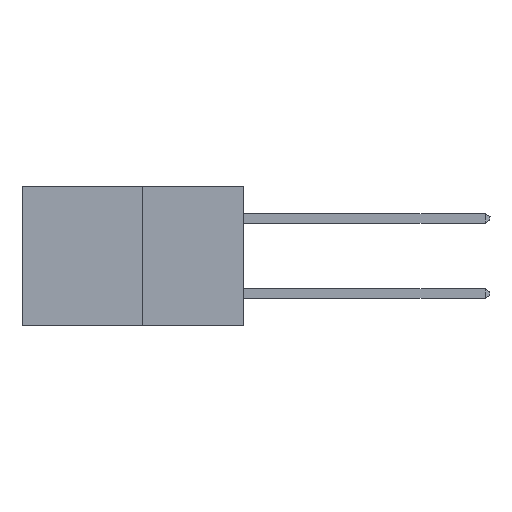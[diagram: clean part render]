
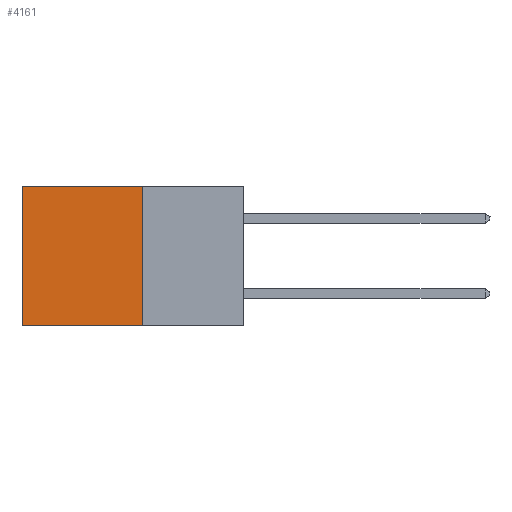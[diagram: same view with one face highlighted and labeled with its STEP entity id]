
A CAD part, left-side view. The second image highlights one B-rep face of the part: STEP entity #4161.
In plain terms, the highlighted planar face has unit normal (-1, 0, 0).
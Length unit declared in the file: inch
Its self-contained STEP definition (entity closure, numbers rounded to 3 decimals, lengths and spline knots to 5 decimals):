
#48 = CARTESIAN_POINT ( 'NONE',  ( 0.277, 0.59, -0.37 ) ) ;
#513 = EDGE_CURVE ( 'NONE', #8192, #10589, #982, .T. ) ;
#982 = LINE ( 'NONE', #8951, #11103 ) ;
#1314 = AXIS2_PLACEMENT_3D ( 'NONE', #7310, #2931, #2757 ) ;
#1714 = EDGE_CURVE ( 'NONE', #8192, #7956, #3690, .T. ) ;
#2119 = CARTESIAN_POINT ( 'NONE',  ( 0.277, 0.27, 0. ) ) ;
#2742 = ORIENTED_EDGE ( 'NONE', *, *, #16108, .T. ) ;
#2757 = DIRECTION ( 'NONE',  ( 0., 0., -1. ) ) ;
#2931 = DIRECTION ( 'NONE',  ( 1., 0., 0. ) ) ;
#3690 = LINE ( 'NONE', #9103, #14407 ) ;
#3857 = CARTESIAN_POINT ( 'NONE',  ( 0.277, 0.59, -0.37 ) ) ;
#4161 = ADVANCED_FACE ( 'NONE', ( #5045 ), #13655, .F. ) ;
#5045 = FACE_OUTER_BOUND ( 'NONE', #12254, .T. ) ;
#5719 = CARTESIAN_POINT ( 'NONE',  ( 0.277, 0.27, -0.37 ) ) ;
#6217 = VECTOR ( 'NONE', #7616, 39.37008 ) ;
#7310 = CARTESIAN_POINT ( 'NONE',  ( 0.277, 0.27, -0.37 ) ) ;
#7616 = DIRECTION ( 'NONE',  ( 0., 1., 0. ) ) ;
#7672 = CARTESIAN_POINT ( 'NONE',  ( 0.277, 0.27, -0.37 ) ) ;
#7956 = VERTEX_POINT ( 'NONE', #7672 ) ;
#8192 = VERTEX_POINT ( 'NONE', #2119 ) ;
#8737 = DIRECTION ( 'NONE',  ( 0., 0., -1. ) ) ;
#8951 = CARTESIAN_POINT ( 'NONE',  ( 0.277, 0.27, 0. ) ) ;
#9103 = CARTESIAN_POINT ( 'NONE',  ( 0.277, 0.27, -0.37 ) ) ;
#9658 = DIRECTION ( 'NONE',  ( 0., 1., 0. ) ) ;
#10034 = DIRECTION ( 'NONE',  ( 0., 0., -1. ) ) ;
#10190 = VERTEX_POINT ( 'NONE', #3857 ) ;
#10589 = VERTEX_POINT ( 'NONE', #14653 ) ;
#10743 = VECTOR ( 'NONE', #10034, 39.37008 ) ;
#11103 = VECTOR ( 'NONE', #9658, 39.37008 ) ;
#11401 = ORIENTED_EDGE ( 'NONE', *, *, #1714, .F. ) ;
#11802 = ORIENTED_EDGE ( 'NONE', *, *, #11987, .F. ) ;
#11987 = EDGE_CURVE ( 'NONE', #7956, #10190, #16237, .T. ) ;
#12254 = EDGE_LOOP ( 'NONE', ( #2742, #11802, #11401, #13370 ) ) ;
#13370 = ORIENTED_EDGE ( 'NONE', *, *, #513, .T. ) ;
#13655 = PLANE ( 'NONE',  #1314 ) ;
#14052 = LINE ( 'NONE', #48, #10743 ) ;
#14407 = VECTOR ( 'NONE', #8737, 39.37008 ) ;
#14653 = CARTESIAN_POINT ( 'NONE',  ( 0.277, 0.59, 0. ) ) ;
#16108 = EDGE_CURVE ( 'NONE', #10589, #10190, #14052, .T. ) ;
#16237 = LINE ( 'NONE', #5719, #6217 ) ;
